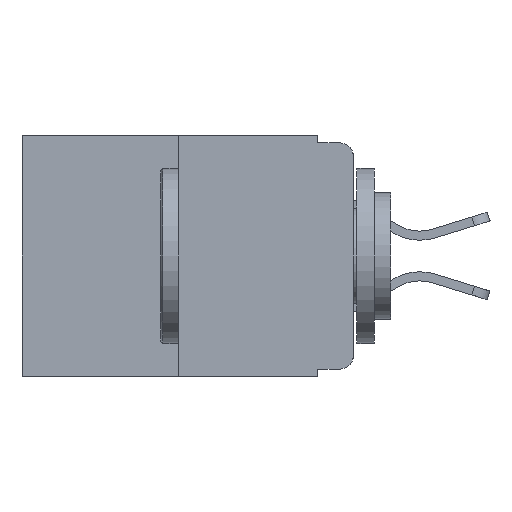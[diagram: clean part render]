
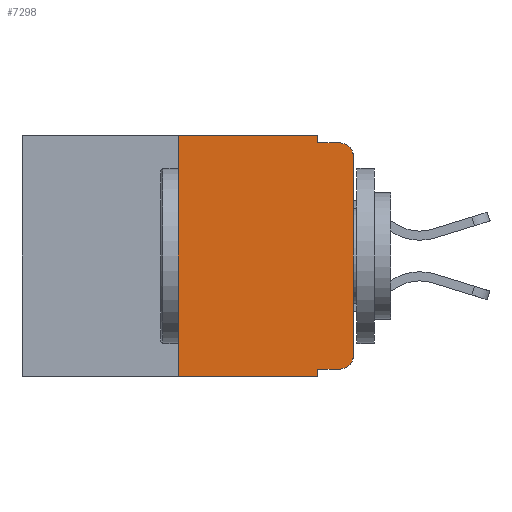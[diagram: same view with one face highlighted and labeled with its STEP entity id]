
A CAD part, left-side view. The second image highlights one B-rep face of the part: STEP entity #7298.
In plain terms, the highlighted planar face has unit normal (-1, 0, 0).
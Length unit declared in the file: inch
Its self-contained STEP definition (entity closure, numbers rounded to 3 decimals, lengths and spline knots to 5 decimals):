
#30 = FACE_OUTER_BOUND ( 'NONE', #5477, .T. ) ;
#112 = VERTEX_POINT ( 'NONE', #878 ) ;
#176 = DIRECTION ( 'NONE',  ( 0., -1., 0. ) ) ;
#356 = ORIENTED_EDGE ( 'NONE', *, *, #4490, .F. ) ;
#404 = LINE ( 'NONE', #3890, #1309 ) ;
#412 = CARTESIAN_POINT ( 'NONE',  ( 0., 0.473, -0.343 ) ) ;
#415 = ORIENTED_EDGE ( 'NONE', *, *, #4024, .T. ) ;
#520 = DIRECTION ( 'NONE',  ( -1., 0., 0. ) ) ;
#878 = CARTESIAN_POINT ( 'NONE',  ( 0., 0.25, -0.343 ) ) ;
#1009 = CARTESIAN_POINT ( 'NONE',  ( 0., 0., -0.313 ) ) ;
#1017 = LINE ( 'NONE', #4450, #3451 ) ;
#1028 = CARTESIAN_POINT ( 'NONE',  ( 0., 0.051, 0. ) ) ;
#1061 = EDGE_CURVE ( 'NONE', #5387, #6232, #404, .T. ) ;
#1072 = CARTESIAN_POINT ( 'NONE',  ( 0., 0.051, -0.343 ) ) ;
#1309 = VECTOR ( 'NONE', #5648, 39.37008 ) ;
#1526 = DIRECTION ( 'NONE',  ( 1., 0., 0. ) ) ;
#1750 = VERTEX_POINT ( 'NONE', #2402 ) ;
#1786 = VECTOR ( 'NONE', #3487, 39.37008 ) ;
#1903 = CARTESIAN_POINT ( 'NONE',  ( 0., 0.051, -0.01 ) ) ;
#2127 = DIRECTION ( 'NONE',  ( 0., 0., -1. ) ) ;
#2133 = DIRECTION ( 'NONE',  ( 0., -1., 0. ) ) ;
#2402 = CARTESIAN_POINT ( 'NONE',  ( 0., 0.02, -0.01 ) ) ;
#2401 = DIRECTION ( 'NONE',  ( 0., 0., -1. ) ) ;
#2560 = VERTEX_POINT ( 'NONE', #1009 ) ;
#2811 = VECTOR ( 'NONE', #176, 39.37008 ) ;
#3155 = AXIS2_PLACEMENT_3D ( 'NONE', #5743, #3788, #2127 ) ;
#3451 = VECTOR ( 'NONE', #10488, 39.37008 ) ;
#3466 = VECTOR ( 'NONE', #2133, 39.37008 ) ;
#3487 = DIRECTION ( 'NONE',  ( 0., 0., -1. ) ) ;
#3593 = LINE ( 'NONE', #6988, #9358 ) ;
#3741 = ORIENTED_EDGE ( 'NONE', *, *, #10478, .T. ) ;
#3788 = DIRECTION ( 'NONE',  ( -1., 0., 0. ) ) ;
#3871 = DIRECTION ( 'NONE',  ( 0., -1., 0. ) ) ;
#3890 = CARTESIAN_POINT ( 'NONE',  ( 0., 0.473, 0. ) ) ;
#4024 = EDGE_CURVE ( 'NONE', #112, #7622, #9253, .T. ) ;
#4055 = CIRCLE ( 'NONE', #3155, 0.02 ) ;
#4395 = LINE ( 'NONE', #1903, #3466 ) ;
#4450 = CARTESIAN_POINT ( 'NONE',  ( 0., 0.25, 0. ) ) ;
#4490 = EDGE_CURVE ( 'NONE', #6232, #7531, #10275, .T. ) ;
#4517 = CARTESIAN_POINT ( 'NONE',  ( 0., 0.051, 0. ) ) ;
#4538 = LINE ( 'NONE', #10750, #10385 ) ;
#4699 = VECTOR ( 'NONE', #3871, 39.37008 ) ;
#4721 = ORIENTED_EDGE ( 'NONE', *, *, #5090, .F. ) ;
#4762 = CARTESIAN_POINT ( 'NONE',  ( 0., 0.25, 0. ) ) ;
#5090 = EDGE_CURVE ( 'NONE', #7531, #1750, #4395, .T. ) ;
#5387 = VERTEX_POINT ( 'NONE', #4762 ) ;
#5477 = EDGE_LOOP ( 'NONE', ( #3741, #7980, #4721, #356, #6157, #9826, #415, #7132, #10386, #10923 ) ) ;
#5590 = CARTESIAN_POINT ( 'NONE',  ( 0., 0.051, -0.333 ) ) ;
#5592 = CARTESIAN_POINT ( 'NONE',  ( 0., 0.02, -0.313 ) ) ;
#5648 = DIRECTION ( 'NONE',  ( 0., -1., 0. ) ) ;
#5701 = DIRECTION ( 'NONE',  ( 0., 0., -1. ) ) ;
#5743 = CARTESIAN_POINT ( 'NONE',  ( 0., 0.02, -0.03 ) ) ;
#6015 = VERTEX_POINT ( 'NONE', #8270 ) ;
#6084 = DIRECTION ( 'NONE',  ( 0., 0., 1. ) ) ;
#6157 = ORIENTED_EDGE ( 'NONE', *, *, #1061, .F. ) ;
#6232 = VERTEX_POINT ( 'NONE', #4517 ) ;
#6454 = EDGE_CURVE ( 'NONE', #9183, #7988, #7076, .T. ) ;
#6663 = CIRCLE ( 'NONE', #10414, 0.02 ) ;
#6906 = EDGE_CURVE ( 'NONE', #9183, #7622, #4538, .T. ) ;
#6926 = CARTESIAN_POINT ( 'NONE',  ( 0., 0.051, -0.333 ) ) ;
#6988 = CARTESIAN_POINT ( 'NONE',  ( 0., 0., 0. ) ) ;
#7076 = LINE ( 'NONE', #6926, #2811 ) ;
#7132 = ORIENTED_EDGE ( 'NONE', *, *, #6906, .F. ) ;
#7298 = ADVANCED_FACE ( 'NONE', ( #30 ), #9240, .F. ) ;
#7531 = VERTEX_POINT ( 'NONE', #7846 ) ;
#7622 = VERTEX_POINT ( 'NONE', #1072 ) ;
#7846 = CARTESIAN_POINT ( 'NONE',  ( 0., 0.051, -0.01 ) ) ;
#7895 = EDGE_CURVE ( 'NONE', #7988, #2560, #6663, .T. ) ;
#7937 = AXIS2_PLACEMENT_3D ( 'NONE', #9970, #1526, #2401 ) ;
#7980 = ORIENTED_EDGE ( 'NONE', *, *, #10077, .T. ) ;
#7988 = VERTEX_POINT ( 'NONE', #9266 ) ;
#8270 = CARTESIAN_POINT ( 'NONE',  ( 0., 0., -0.03 ) ) ;
#9183 = VERTEX_POINT ( 'NONE', #5590 ) ;
#9240 = PLANE ( 'NONE',  #7937 ) ;
#9253 = LINE ( 'NONE', #412, #4699 ) ;
#9266 = CARTESIAN_POINT ( 'NONE',  ( 0., 0.02, -0.333 ) ) ;
#9358 = VECTOR ( 'NONE', #6084, 39.37008 ) ;
#9665 = EDGE_CURVE ( 'NONE', #112, #5387, #1017, .T. ) ;
#9826 = ORIENTED_EDGE ( 'NONE', *, *, #9665, .F. ) ;
#9863 = DIRECTION ( 'NONE',  ( 0., 0., -1. ) ) ;
#9970 = CARTESIAN_POINT ( 'NONE',  ( 0., 0.473, 0. ) ) ;
#10077 = EDGE_CURVE ( 'NONE', #6015, #1750, #4055, .T. ) ;
#10275 = LINE ( 'NONE', #1028, #1786 ) ;
#10385 = VECTOR ( 'NONE', #9863, 39.37008 ) ;
#10386 = ORIENTED_EDGE ( 'NONE', *, *, #6454, .T. ) ;
#10414 = AXIS2_PLACEMENT_3D ( 'NONE', #5592, #520, #5701 ) ;
#10478 = EDGE_CURVE ( 'NONE', #2560, #6015, #3593, .T. ) ;
#10488 = DIRECTION ( 'NONE',  ( 0., 0., 1. ) ) ;
#10750 = CARTESIAN_POINT ( 'NONE',  ( 0., 0.051, 0. ) ) ;
#10923 = ORIENTED_EDGE ( 'NONE', *, *, #7895, .T. ) ;
